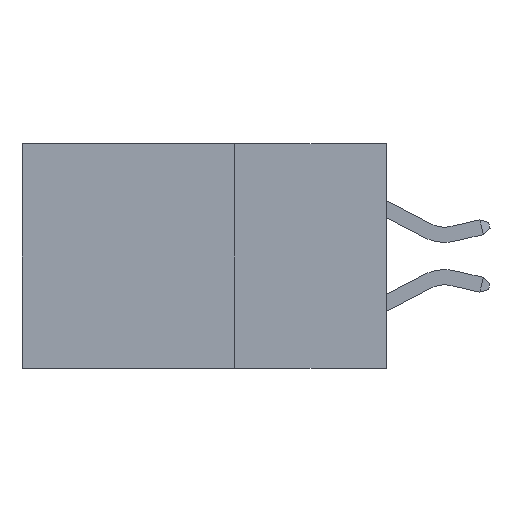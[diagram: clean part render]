
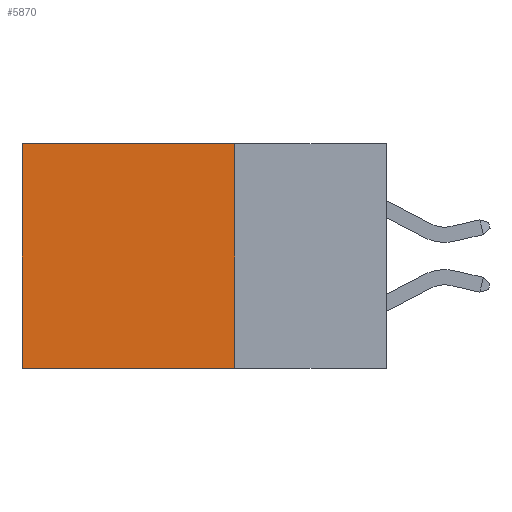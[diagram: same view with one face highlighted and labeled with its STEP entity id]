
A CAD part, left-side view. The second image highlights one B-rep face of the part: STEP entity #5870.
In plain terms, the highlighted planar face has unit normal (-1, 0, 0).
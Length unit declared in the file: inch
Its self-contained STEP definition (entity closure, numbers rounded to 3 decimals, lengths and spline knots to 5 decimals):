
#32 = DIRECTION ( 'NONE',  ( 0., 0., -1. ) ) ;
#1189 = EDGE_CURVE ( 'NONE', #11351, #21767, #1310, .T. ) ;
#1310 = LINE ( 'NONE', #8479, #4444 ) ;
#1427 = ORIENTED_EDGE ( 'NONE', *, *, #1189, .F. ) ;
#2345 = CARTESIAN_POINT ( 'NONE',  ( 0.2615, 0.6, -0.37 ) ) ;
#2801 = CARTESIAN_POINT ( 'NONE',  ( 0.2615, 0.6, 0. ) ) ;
#3101 = VECTOR ( 'NONE', #4003, 39.37008 ) ;
#3306 = CARTESIAN_POINT ( 'NONE',  ( 0.2615, 0.25, -0.37 ) ) ;
#3786 = CARTESIAN_POINT ( 'NONE',  ( 0.2615, 0.25, 0. ) ) ;
#4003 = DIRECTION ( 'NONE',  ( 0., 0., -1. ) ) ;
#4444 = VECTOR ( 'NONE', #4764, 39.37008 ) ;
#4704 = DIRECTION ( 'NONE',  ( 0., 1., 0. ) ) ;
#4764 = DIRECTION ( 'NONE',  ( 0., 0., -1. ) ) ;
#5870 = ADVANCED_FACE ( 'NONE', ( #15305 ), #21881, .F. ) ;
#6632 = CARTESIAN_POINT ( 'NONE',  ( 0.2615, 0.25, -0.37 ) ) ;
#6849 = VECTOR ( 'NONE', #4704, 39.37008 ) ;
#8479 = CARTESIAN_POINT ( 'NONE',  ( 0.2615, 0.25, -0.37 ) ) ;
#9072 = ORIENTED_EDGE ( 'NONE', *, *, #10514, .F. ) ;
#9819 = EDGE_LOOP ( 'NONE', ( #15095, #9072, #1427, #18793 ) ) ;
#10514 = EDGE_CURVE ( 'NONE', #21767, #17341, #13240, .T. ) ;
#10993 = EDGE_CURVE ( 'NONE', #11351, #14848, #19938, .T. ) ;
#11315 = CARTESIAN_POINT ( 'NONE',  ( 0.2615, 0.25, 0. ) ) ;
#11351 = VERTEX_POINT ( 'NONE', #3786 ) ;
#12542 = CARTESIAN_POINT ( 'NONE',  ( 0.2615, 0.6, -0.37 ) ) ;
#13240 = LINE ( 'NONE', #20069, #6849 ) ;
#13375 = DIRECTION ( 'NONE',  ( 1., 0., 0. ) ) ;
#14416 = VECTOR ( 'NONE', #21516, 39.37008 ) ;
#14848 = VERTEX_POINT ( 'NONE', #2801 ) ;
#15095 = ORIENTED_EDGE ( 'NONE', *, *, #21521, .T. ) ;
#15305 = FACE_OUTER_BOUND ( 'NONE', #9819, .T. ) ;
#15908 = LINE ( 'NONE', #12542, #3101 ) ;
#17341 = VERTEX_POINT ( 'NONE', #2345 ) ;
#18793 = ORIENTED_EDGE ( 'NONE', *, *, #10993, .T. ) ;
#19938 = LINE ( 'NONE', #11315, #14416 ) ;
#20069 = CARTESIAN_POINT ( 'NONE',  ( 0.2615, 0.25, -0.37 ) ) ;
#21302 = AXIS2_PLACEMENT_3D ( 'NONE', #6632, #13375, #32 ) ;
#21516 = DIRECTION ( 'NONE',  ( 0., 1., 0. ) ) ;
#21521 = EDGE_CURVE ( 'NONE', #14848, #17341, #15908, .T. ) ;
#21767 = VERTEX_POINT ( 'NONE', #3306 ) ;
#21881 = PLANE ( 'NONE',  #21302 ) ;
